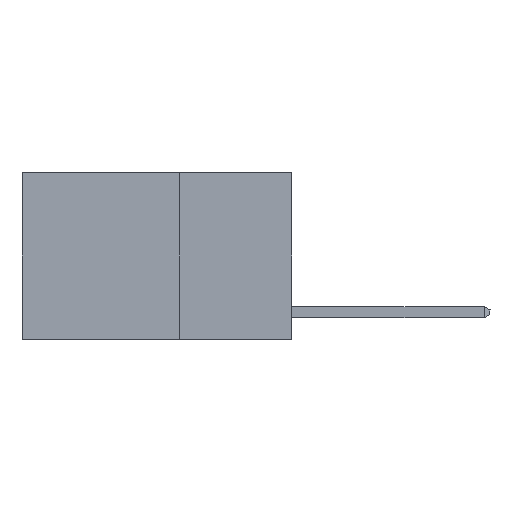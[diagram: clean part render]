
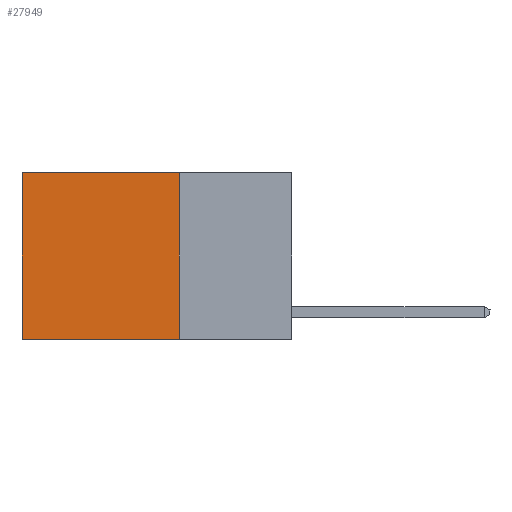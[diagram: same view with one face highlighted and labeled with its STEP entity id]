
A CAD part, left-side view. The second image highlights one B-rep face of the part: STEP entity #27949.
In plain terms, the highlighted planar face has unit normal (-1, 0, 0).
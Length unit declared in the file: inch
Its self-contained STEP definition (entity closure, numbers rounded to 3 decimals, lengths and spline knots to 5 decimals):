
#112 = VECTOR ( 'NONE', #13312, 39.37008 ) ;
#184 = CARTESIAN_POINT ( 'NONE',  ( 0.2625, 0.25, 0. ) ) ;
#416 = CARTESIAN_POINT ( 'NONE',  ( 0.2625, 0.25, 0. ) ) ;
#660 = DIRECTION ( 'NONE',  ( 1., 0., 0. ) ) ;
#2832 = EDGE_LOOP ( 'NONE', ( #27867, #5851, #26106, #20313 ) ) ;
#5851 = ORIENTED_EDGE ( 'NONE', *, *, #16757, .F. ) ;
#7608 = DIRECTION ( 'NONE',  ( 0., 1., 0. ) ) ;
#8094 = LINE ( 'NONE', #416, #24638 ) ;
#11144 = VERTEX_POINT ( 'NONE', #24622 ) ;
#11502 = LINE ( 'NONE', #12870, #22313 ) ;
#11712 = EDGE_CURVE ( 'NONE', #11144, #23655, #8094, .T. ) ;
#12316 = FACE_OUTER_BOUND ( 'NONE', #2832, .T. ) ;
#12870 = CARTESIAN_POINT ( 'NONE',  ( 0.2625, 0.6, 0. ) ) ;
#13312 = DIRECTION ( 'NONE',  ( 0., 1., 0. ) ) ;
#13690 = CARTESIAN_POINT ( 'NONE',  ( 0.2625, 0.25, 0. ) ) ;
#13878 = EDGE_CURVE ( 'NONE', #11144, #26391, #23194, .T. ) ;
#14293 = LINE ( 'NONE', #18400, #25750 ) ;
#15628 = DIRECTION ( 'NONE',  ( 0., 0., -1. ) ) ;
#15849 = DIRECTION ( 'NONE',  ( 0., 0., -1. ) ) ;
#16757 = EDGE_CURVE ( 'NONE', #23655, #22176, #14293, .T. ) ;
#17093 = CARTESIAN_POINT ( 'NONE',  ( 0.2625, 0.6, 0. ) ) ;
#17736 = EDGE_CURVE ( 'NONE', #26391, #22176, #11502, .T. ) ;
#18400 = CARTESIAN_POINT ( 'NONE',  ( 0.2625, 0.25, -0.37 ) ) ;
#19057 = AXIS2_PLACEMENT_3D ( 'NONE', #13690, #660, #15849 ) ;
#19394 = DIRECTION ( 'NONE',  ( 0., 0., -1. ) ) ;
#20313 = ORIENTED_EDGE ( 'NONE', *, *, #13878, .T. ) ;
#22176 = VERTEX_POINT ( 'NONE', #22186 ) ;
#22186 = CARTESIAN_POINT ( 'NONE',  ( 0.2625, 0.6, -0.37 ) ) ;
#22266 = PLANE ( 'NONE',  #19057 ) ;
#22313 = VECTOR ( 'NONE', #19394, 39.37008 ) ;
#23194 = LINE ( 'NONE', #184, #112 ) ;
#23655 = VERTEX_POINT ( 'NONE', #27995 ) ;
#24622 = CARTESIAN_POINT ( 'NONE',  ( 0.2625, 0.25, 0. ) ) ;
#24638 = VECTOR ( 'NONE', #15628, 39.37008 ) ;
#25750 = VECTOR ( 'NONE', #7608, 39.37008 ) ;
#26106 = ORIENTED_EDGE ( 'NONE', *, *, #11712, .F. ) ;
#26391 = VERTEX_POINT ( 'NONE', #17093 ) ;
#27867 = ORIENTED_EDGE ( 'NONE', *, *, #17736, .T. ) ;
#27949 = ADVANCED_FACE ( 'NONE', ( #12316 ), #22266, .F. ) ;
#27995 = CARTESIAN_POINT ( 'NONE',  ( 0.2625, 0.25, -0.37 ) ) ;
